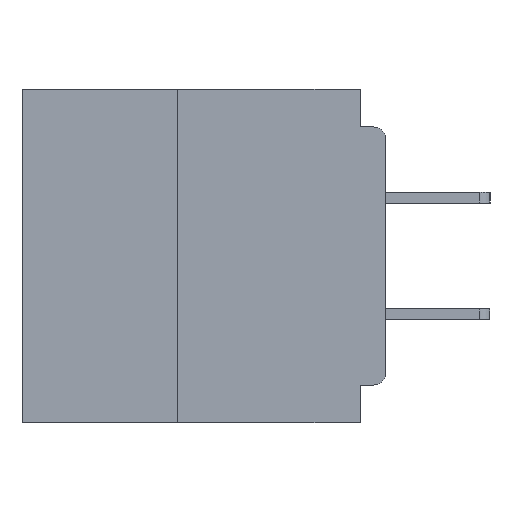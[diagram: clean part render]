
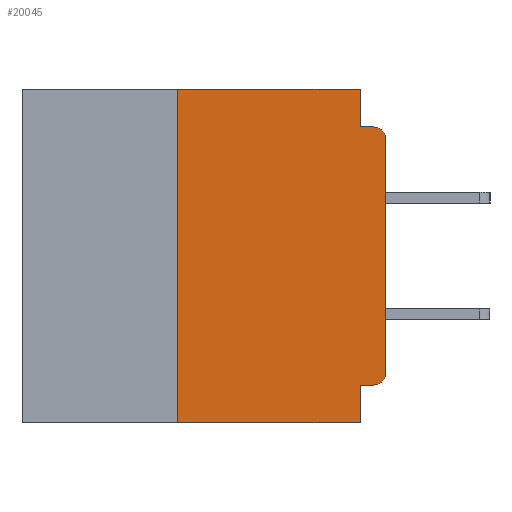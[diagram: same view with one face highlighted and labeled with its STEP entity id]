
A CAD part, left-side view. The second image highlights one B-rep face of the part: STEP entity #20045.
In plain terms, the highlighted planar face has unit normal (-1, 0, 0).
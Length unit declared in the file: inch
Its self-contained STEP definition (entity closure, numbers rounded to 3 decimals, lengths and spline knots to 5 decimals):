
#267 = VECTOR ( 'NONE', #30683, 39.37008 ) ;
#400 = ORIENTED_EDGE ( 'NONE', *, *, #39247, .T. ) ;
#545 = CARTESIAN_POINT ( 'NONE',  ( 0., 0.015, -0.34 ) ) ;
#732 = LINE ( 'NONE', #37317, #39990 ) ;
#983 = CARTESIAN_POINT ( 'NONE',  ( 0., 0.031, -0.4 ) ) ;
#1357 = PLANE ( 'NONE',  #34855 ) ;
#1691 = VERTEX_POINT ( 'NONE', #33692 ) ;
#3288 = EDGE_LOOP ( 'NONE', ( #17803, #19724, #14842, #25351, #39537, #38037, #12615, #13339, #31187, #400 ) ) ;
#3612 = LINE ( 'NONE', #12143, #35585 ) ;
#3710 = DIRECTION ( 'NONE',  ( 0., 0., -1. ) ) ;
#4098 = DIRECTION ( 'NONE',  ( 0., 0., -1. ) ) ;
#4511 = DIRECTION ( 'NONE',  ( 0., 0., -1. ) ) ;
#4926 = DIRECTION ( 'NONE',  ( 0., -1., 0. ) ) ;
#5488 = VECTOR ( 'NONE', #4098, 39.37008 ) ;
#6739 = DIRECTION ( 'NONE',  ( 0., 0., 1. ) ) ;
#7266 = EDGE_CURVE ( 'NONE', #23386, #17721, #23520, .T. ) ;
#7335 = DIRECTION ( 'NONE',  ( 0., 0., -1. ) ) ;
#7744 = CARTESIAN_POINT ( 'NONE',  ( 0., 0.25, -0.4 ) ) ;
#8030 = DIRECTION ( 'NONE',  ( -1., 0., 0. ) ) ;
#8035 = CARTESIAN_POINT ( 'NONE',  ( 0., 0.015, -0.355 ) ) ;
#8052 = VERTEX_POINT ( 'NONE', #19828 ) ;
#9130 = DIRECTION ( 'NONE',  ( 0., 0., 1. ) ) ;
#10322 = CARTESIAN_POINT ( 'NONE',  ( 0., 0.031, -0.045 ) ) ;
#11421 = CARTESIAN_POINT ( 'NONE',  ( 0., 0., -0.34 ) ) ;
#12139 = CIRCLE ( 'NONE', #21808, 0.015 ) ;
#12143 = CARTESIAN_POINT ( 'NONE',  ( 0., 0., 0. ) ) ;
#12255 = VERTEX_POINT ( 'NONE', #8035 ) ;
#12461 = DIRECTION ( 'NONE',  ( 0., -1., 0. ) ) ;
#12615 = ORIENTED_EDGE ( 'NONE', *, *, #7266, .T. ) ;
#13163 = CARTESIAN_POINT ( 'NONE',  ( 0., 0.031, -0.355 ) ) ;
#13339 = ORIENTED_EDGE ( 'NONE', *, *, #36864, .F. ) ;
#13827 = LINE ( 'NONE', #25750, #5488 ) ;
#13837 = CARTESIAN_POINT ( 'NONE',  ( 0., 0.437, 0. ) ) ;
#14142 = EDGE_CURVE ( 'NONE', #14573, #28080, #3612, .T. ) ;
#14573 = VERTEX_POINT ( 'NONE', #11421 ) ;
#14606 = VECTOR ( 'NONE', #12461, 39.37008 ) ;
#14842 = ORIENTED_EDGE ( 'NONE', *, *, #26092, .F. ) ;
#14978 = EDGE_CURVE ( 'NONE', #8052, #31087, #13827, .T. ) ;
#15603 = LINE ( 'NONE', #24781, #14606 ) ;
#16369 = EDGE_CURVE ( 'NONE', #23386, #38494, #31347, .T. ) ;
#16961 = LINE ( 'NONE', #36823, #267 ) ;
#17721 = VERTEX_POINT ( 'NONE', #20213 ) ;
#17803 = ORIENTED_EDGE ( 'NONE', *, *, #14142, .T. ) ;
#18142 = VERTEX_POINT ( 'NONE', #13163 ) ;
#19724 = ORIENTED_EDGE ( 'NONE', *, *, #26473, .T. ) ;
#19828 = CARTESIAN_POINT ( 'NONE',  ( 0., 0.031, 0. ) ) ;
#20045 = ADVANCED_FACE ( 'NONE', ( #32457 ), #1357, .F. ) ;
#20213 = CARTESIAN_POINT ( 'NONE',  ( 0., 0.031, -0.4 ) ) ;
#21808 = AXIS2_PLACEMENT_3D ( 'NONE', #545, #22366, #3710 ) ;
#22031 = EDGE_CURVE ( 'NONE', #12255, #18142, #732, .T. ) ;
#22366 = DIRECTION ( 'NONE',  ( -1., 0., 0. ) ) ;
#23140 = DIRECTION ( 'NONE',  ( 1., 0., 0. ) ) ;
#23386 = VERTEX_POINT ( 'NONE', #7744 ) ;
#23520 = LINE ( 'NONE', #26672, #38905 ) ;
#24114 = VECTOR ( 'NONE', #6739, 39.37008 ) ;
#24232 = CARTESIAN_POINT ( 'NONE',  ( 0., 0., -0.06 ) ) ;
#24781 = CARTESIAN_POINT ( 'NONE',  ( 0., 0.437, 0. ) ) ;
#25351 = ORIENTED_EDGE ( 'NONE', *, *, #14978, .F. ) ;
#25750 = CARTESIAN_POINT ( 'NONE',  ( 0., 0.031, 0. ) ) ;
#26092 = EDGE_CURVE ( 'NONE', #31087, #1691, #16961, .T. ) ;
#26473 = EDGE_CURVE ( 'NONE', #28080, #1691, #34809, .T. ) ;
#26597 = CARTESIAN_POINT ( 'NONE',  ( 0., 0.015, -0.06 ) ) ;
#26672 = CARTESIAN_POINT ( 'NONE',  ( 0., 0.437, -0.4 ) ) ;
#28080 = VERTEX_POINT ( 'NONE', #24232 ) ;
#28375 = VECTOR ( 'NONE', #7335, 39.37008 ) ;
#28443 = CARTESIAN_POINT ( 'NONE',  ( 0., 0.25, -0.4 ) ) ;
#29705 = DIRECTION ( 'NONE',  ( 0., 0., -1. ) ) ;
#30683 = DIRECTION ( 'NONE',  ( 0., -1., 0. ) ) ;
#31087 = VERTEX_POINT ( 'NONE', #10322 ) ;
#31187 = ORIENTED_EDGE ( 'NONE', *, *, #22031, .F. ) ;
#31309 = DIRECTION ( 'NONE',  ( 0., 1., 0. ) ) ;
#31347 = LINE ( 'NONE', #28443, #24114 ) ;
#31537 = EDGE_CURVE ( 'NONE', #38494, #8052, #15603, .T. ) ;
#32457 = FACE_OUTER_BOUND ( 'NONE', #3288, .T. ) ;
#33692 = CARTESIAN_POINT ( 'NONE',  ( 0., 0.015, -0.045 ) ) ;
#34809 = CIRCLE ( 'NONE', #35239, 0.015 ) ;
#34855 = AXIS2_PLACEMENT_3D ( 'NONE', #13837, #23140, #4511 ) ;
#35239 = AXIS2_PLACEMENT_3D ( 'NONE', #26597, #8030, #29705 ) ;
#35585 = VECTOR ( 'NONE', #9130, 39.37008 ) ;
#36499 = LINE ( 'NONE', #983, #28375 ) ;
#36823 = CARTESIAN_POINT ( 'NONE',  ( 0., 0., -0.045 ) ) ;
#36864 = EDGE_CURVE ( 'NONE', #18142, #17721, #36499, .T. ) ;
#36944 = CARTESIAN_POINT ( 'NONE',  ( 0., 0.25, 0. ) ) ;
#37317 = CARTESIAN_POINT ( 'NONE',  ( 0., 0., -0.355 ) ) ;
#38037 = ORIENTED_EDGE ( 'NONE', *, *, #16369, .F. ) ;
#38494 = VERTEX_POINT ( 'NONE', #36944 ) ;
#38905 = VECTOR ( 'NONE', #4926, 39.37008 ) ;
#39247 = EDGE_CURVE ( 'NONE', #12255, #14573, #12139, .T. ) ;
#39537 = ORIENTED_EDGE ( 'NONE', *, *, #31537, .F. ) ;
#39990 = VECTOR ( 'NONE', #31309, 39.37008 ) ;
